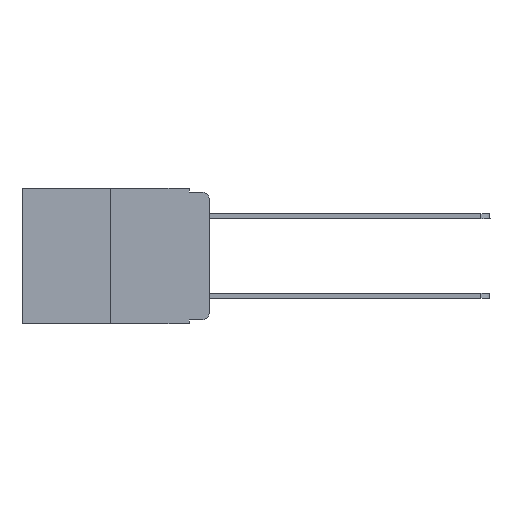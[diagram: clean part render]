
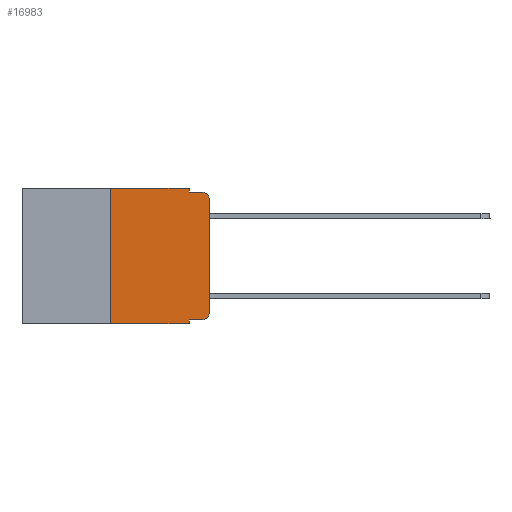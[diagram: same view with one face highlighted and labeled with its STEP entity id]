
A CAD part, left-side view. The second image highlights one B-rep face of the part: STEP entity #16983.
In plain terms, the highlighted planar face has unit normal (-1, 0, 0).
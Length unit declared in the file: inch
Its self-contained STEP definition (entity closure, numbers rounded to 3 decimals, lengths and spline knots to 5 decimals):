
#193 = CARTESIAN_POINT ( 'NONE',  ( 0., 0.051, 0. ) ) ;
#353 = CARTESIAN_POINT ( 'NONE',  ( 0., 0.02, -0.01 ) ) ;
#411 = ORIENTED_EDGE ( 'NONE', *, *, #5507, .F. ) ;
#633 = DIRECTION ( 'NONE',  ( 0., -1., 0. ) ) ;
#644 = EDGE_CURVE ( 'NONE', #1210, #8631, #8910, .T. ) ;
#927 = ORIENTED_EDGE ( 'NONE', *, *, #12250, .T. ) ;
#1123 = CARTESIAN_POINT ( 'NONE',  ( 0., 0.473, 0. ) ) ;
#1160 = LINE ( 'NONE', #7112, #12680 ) ;
#1210 = VERTEX_POINT ( 'NONE', #5347 ) ;
#1576 = ORIENTED_EDGE ( 'NONE', *, *, #8611, .F. ) ;
#1759 = EDGE_CURVE ( 'NONE', #8631, #10914, #3721, .T. ) ;
#1878 = EDGE_CURVE ( 'NONE', #2893, #17008, #7413, .T. ) ;
#2048 = VECTOR ( 'NONE', #10673, 39.37008 ) ;
#2441 = CARTESIAN_POINT ( 'NONE',  ( 0., 0.051, -0.333 ) ) ;
#2727 = VECTOR ( 'NONE', #16954, 39.37008 ) ;
#2802 = LINE ( 'NONE', #2441, #6130 ) ;
#2893 = VERTEX_POINT ( 'NONE', #11075 ) ;
#3008 = LINE ( 'NONE', #4427, #16561 ) ;
#3257 = AXIS2_PLACEMENT_3D ( 'NONE', #4257, #9520, #16216 ) ;
#3721 = LINE ( 'NONE', #193, #2048 ) ;
#3764 = EDGE_CURVE ( 'NONE', #16313, #2893, #2802, .T. ) ;
#3868 = LINE ( 'NONE', #13866, #4079 ) ;
#4047 = AXIS2_PLACEMENT_3D ( 'NONE', #13212, #14532, #15776 ) ;
#4079 = VECTOR ( 'NONE', #633, 39.37008 ) ;
#4084 = ORIENTED_EDGE ( 'NONE', *, *, #644, .F. ) ;
#4257 = CARTESIAN_POINT ( 'NONE',  ( 0., 0.02, -0.313 ) ) ;
#4427 = CARTESIAN_POINT ( 'NONE',  ( 0., 0.051, -0.01 ) ) ;
#4623 = DIRECTION ( 'NONE',  ( 1., 0., 0. ) ) ;
#5347 = CARTESIAN_POINT ( 'NONE',  ( 0., 0.25, 0. ) ) ;
#5507 = EDGE_CURVE ( 'NONE', #10914, #8501, #3008, .T. ) ;
#5845 = CARTESIAN_POINT ( 'NONE',  ( 0., 0., -0.313 ) ) ;
#6015 = CARTESIAN_POINT ( 'NONE',  ( 0., 0.473, 0. ) ) ;
#6130 = VECTOR ( 'NONE', #14332, 39.37008 ) ;
#6135 = CARTESIAN_POINT ( 'NONE',  ( 0., 0.25, 0. ) ) ;
#6308 = ORIENTED_EDGE ( 'NONE', *, *, #12075, .T. ) ;
#7112 = CARTESIAN_POINT ( 'NONE',  ( 0., 0., 0. ) ) ;
#7180 = DIRECTION ( 'NONE',  ( 0., -1., 0. ) ) ;
#7413 = CIRCLE ( 'NONE', #3257, 0.02 ) ;
#7419 = CARTESIAN_POINT ( 'NONE',  ( 0., 0.25, -0.343 ) ) ;
#7883 = VERTEX_POINT ( 'NONE', #11647 ) ;
#7886 = ORIENTED_EDGE ( 'NONE', *, *, #8801, .F. ) ;
#8084 = CARTESIAN_POINT ( 'NONE',  ( 0., 0.051, -0.01 ) ) ;
#8501 = VERTEX_POINT ( 'NONE', #353 ) ;
#8520 = DIRECTION ( 'NONE',  ( 0., 0., -1. ) ) ;
#8611 = EDGE_CURVE ( 'NONE', #9050, #1210, #8707, .T. ) ;
#8631 = VERTEX_POINT ( 'NONE', #9110 ) ;
#8707 = LINE ( 'NONE', #6135, #10126 ) ;
#8801 = EDGE_CURVE ( 'NONE', #16313, #16239, #9314, .T. ) ;
#8910 = LINE ( 'NONE', #1123, #2727 ) ;
#9050 = VERTEX_POINT ( 'NONE', #7419 ) ;
#9110 = CARTESIAN_POINT ( 'NONE',  ( 0., 0.051, 0. ) ) ;
#9314 = LINE ( 'NONE', #13504, #14854 ) ;
#9520 = DIRECTION ( 'NONE',  ( -1., 0., 0. ) ) ;
#9545 = DIRECTION ( 'NONE',  ( 0., 0., -1. ) ) ;
#9973 = EDGE_LOOP ( 'NONE', ( #6308, #14410, #411, #11815, #4084, #1576, #927, #7886, #13330, #15553 ) ) ;
#10126 = VECTOR ( 'NONE', #13855, 39.37008 ) ;
#10480 = CIRCLE ( 'NONE', #4047, 0.02 ) ;
#10673 = DIRECTION ( 'NONE',  ( 0., 0., -1. ) ) ;
#10871 = EDGE_CURVE ( 'NONE', #7883, #8501, #10480, .T. ) ;
#10914 = VERTEX_POINT ( 'NONE', #8084 ) ;
#11075 = CARTESIAN_POINT ( 'NONE',  ( 0., 0.02, -0.333 ) ) ;
#11476 = FACE_OUTER_BOUND ( 'NONE', #9973, .T. ) ;
#11647 = CARTESIAN_POINT ( 'NONE',  ( 0., 0., -0.03 ) ) ;
#11815 = ORIENTED_EDGE ( 'NONE', *, *, #1759, .F. ) ;
#12075 = EDGE_CURVE ( 'NONE', #17008, #7883, #1160, .T. ) ;
#12250 = EDGE_CURVE ( 'NONE', #9050, #16239, #3868, .T. ) ;
#12317 = DIRECTION ( 'NONE',  ( 0., 0., 1. ) ) ;
#12680 = VECTOR ( 'NONE', #12317, 39.37008 ) ;
#13212 = CARTESIAN_POINT ( 'NONE',  ( 0., 0.02, -0.03 ) ) ;
#13330 = ORIENTED_EDGE ( 'NONE', *, *, #3764, .T. ) ;
#13504 = CARTESIAN_POINT ( 'NONE',  ( 0., 0.051, 0. ) ) ;
#13855 = DIRECTION ( 'NONE',  ( 0., 0., 1. ) ) ;
#13866 = CARTESIAN_POINT ( 'NONE',  ( 0., 0.473, -0.343 ) ) ;
#14332 = DIRECTION ( 'NONE',  ( 0., -1., 0. ) ) ;
#14410 = ORIENTED_EDGE ( 'NONE', *, *, #10871, .T. ) ;
#14532 = DIRECTION ( 'NONE',  ( -1., 0., 0. ) ) ;
#14650 = CARTESIAN_POINT ( 'NONE',  ( 0., 0.051, -0.333 ) ) ;
#14854 = VECTOR ( 'NONE', #9545, 39.37008 ) ;
#15553 = ORIENTED_EDGE ( 'NONE', *, *, #1878, .T. ) ;
#15617 = CARTESIAN_POINT ( 'NONE',  ( 0., 0.051, -0.343 ) ) ;
#15776 = DIRECTION ( 'NONE',  ( 0., 0., -1. ) ) ;
#16174 = AXIS2_PLACEMENT_3D ( 'NONE', #6015, #4623, #8520 ) ;
#16216 = DIRECTION ( 'NONE',  ( 0., 0., -1. ) ) ;
#16239 = VERTEX_POINT ( 'NONE', #15617 ) ;
#16313 = VERTEX_POINT ( 'NONE', #14650 ) ;
#16403 = PLANE ( 'NONE',  #16174 ) ;
#16561 = VECTOR ( 'NONE', #7180, 39.37008 ) ;
#16954 = DIRECTION ( 'NONE',  ( 0., -1., 0. ) ) ;
#16983 = ADVANCED_FACE ( 'NONE', ( #11476 ), #16403, .F. ) ;
#17008 = VERTEX_POINT ( 'NONE', #5845 ) ;
